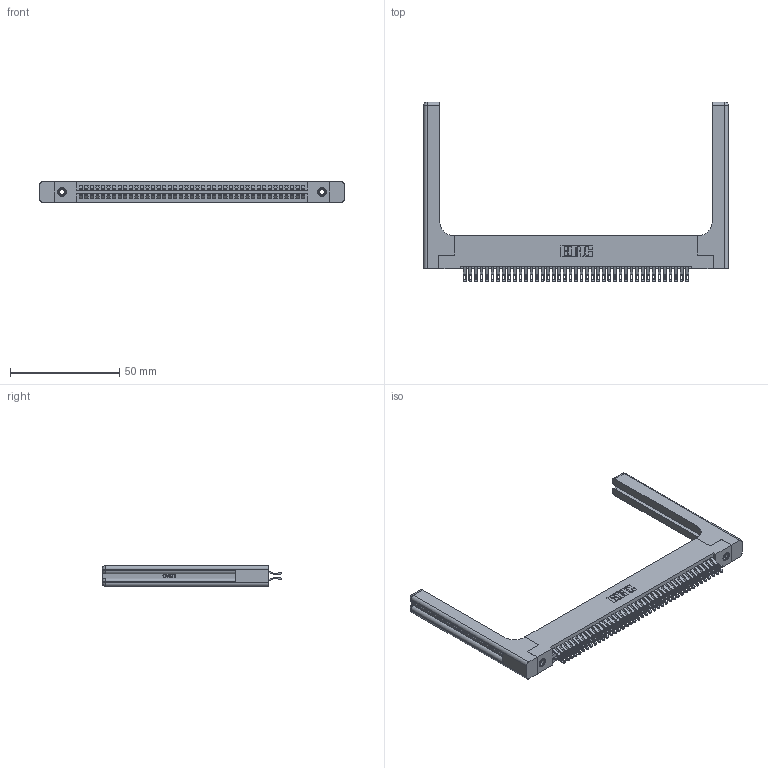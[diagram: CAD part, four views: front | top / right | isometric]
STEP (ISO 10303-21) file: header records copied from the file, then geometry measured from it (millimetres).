
FILE_DESCRIPTION (( 'STEP AP203' ), '1' );
FILE_NAME ('395-082-555-258.STEP', '2019-10-25T07:08:34', ( '' ), ( '' ), 'SwSTEP 2.0', 'SolidWorks 2016', '' );
FILE_SCHEMA (( 'CONFIG_CONTROL_DESIGN' ));
Length unit declared in the file: inch
Products named in the file (5): 345 Part_Flush Mounting Lugs - 0.156 Dia-TH; 345-292-001_555 Tail; 345-250-001_345-250-001-102; 345-220-058_345-220-058; 395-082-555-258
Assembly tree (87 placements, depth 2):
  395-082-555-258
    345 Part_Flush Mounting Lugs - 0.156 Dia-TH
    345-292-001_555 Tail  x82
    345-250-001_345-250-001-102  x2
    345-220-058_345-220-058  x2
Bounding box: 139.17 x 82.09 x 9.4 mm (x, y, z)
Volume: 22222.5 mm3; surface area: 26187.6 mm2
Topology: 87 solids, 87 shells, 4974 faces, 15521 edges, 10326 vertices
Faces by surface type: plane 2770, cylinder 2144, bspline 36, cone 12, sphere 8, torus 4
Entity records: 37812 total; most frequent: CARTESIAN_POINT 7367, ORIENTED_EDGE 6068, DIRECTION 5398, EDGE_CURVE 3034, LINE 2626, VECTOR 2626, VERTEX_POINT 2014, AXIS2_PLACEMENT_3D 1386
